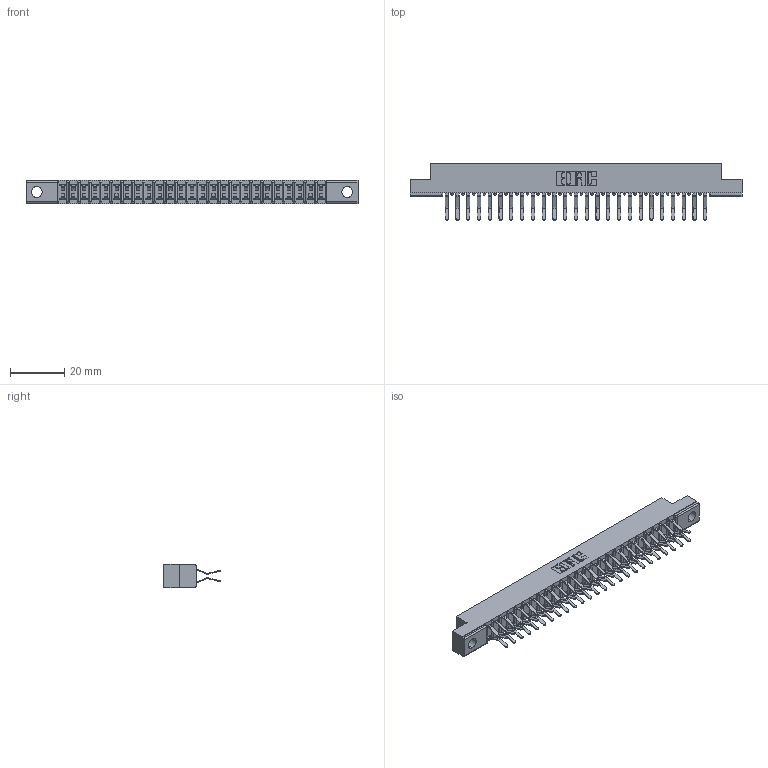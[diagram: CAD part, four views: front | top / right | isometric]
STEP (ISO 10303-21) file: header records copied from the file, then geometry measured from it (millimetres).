
FILE_DESCRIPTION (( 'STEP AP203' ), '1' );
FILE_NAME ('357-050-460-204.STEP', '2020-10-04T06:23:11', ( '' ), ( '' ), 'SwSTEP 2.0', 'SolidWorks 2020', '' );
FILE_SCHEMA (( 'CONFIG_CONTROL_DESIGN' ));
Length unit declared in the file: inch
Products named in the file (3): 307 Part_.156 Dia Mounting Holes; 357-050-460-204; 307-290-001_560
Assembly tree (51 placements, depth 2):
  357-050-460-204
    307 Part_.156 Dia Mounting Holes
    307-290-001_560  x50
Bounding box: 122.07 x 20.73 x 8.71 mm (x, y, z)
Volume: 7940.9 mm3; surface area: 14448.9 mm2
Topology: 51 solids, 51 shells, 2658 faces, 7459 edges, 4834 vertices
Faces by surface type: plane 1734, cylinder 872, sphere 52
Entity records: 24850 total; most frequent: CARTESIAN_POINT 4075, ORIENTED_EDGE 4034, DIRECTION 3991, EDGE_CURVE 2017, LINE 1547, VECTOR 1547, VERTEX_POINT 1306, AXIS2_PLACEMENT_3D 1222
